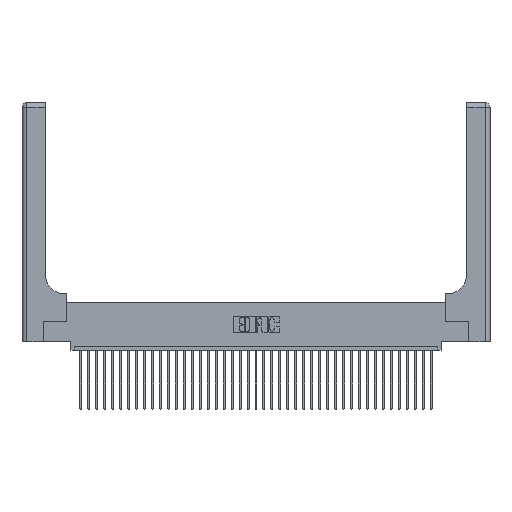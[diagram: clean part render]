
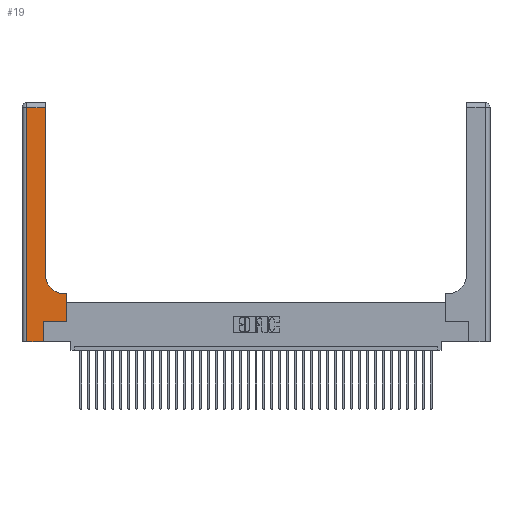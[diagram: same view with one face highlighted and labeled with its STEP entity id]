
A CAD part, top view. The second image highlights one B-rep face of the part: STEP entity #19.
In plain terms, the highlighted planar face has unit normal (0, 0, 1).
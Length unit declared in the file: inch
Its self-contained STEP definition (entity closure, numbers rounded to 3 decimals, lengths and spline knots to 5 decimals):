
#19 = ADVANCED_FACE ( 'NONE', ( #24024 ), #33489, .F. ) ;
#520 = CIRCLE ( 'NONE', #33592, 0.25 ) ;
#1753 = DIRECTION ( 'NONE',  ( 0., 1., 0. ) ) ;
#1925 = EDGE_CURVE ( 'NONE', #36288, #33440, #13026, .T. ) ;
#2226 = ORIENTED_EDGE ( 'NONE', *, *, #29808, .T. ) ;
#2275 = ORIENTED_EDGE ( 'NONE', *, *, #37258, .T. ) ;
#2957 = CARTESIAN_POINT ( 'NONE',  ( 0.2915, 2.94, 0.37 ) ) ;
#3867 = DIRECTION ( 'NONE',  ( 0., -1., 0. ) ) ;
#3986 = CARTESIAN_POINT ( 'NONE',  ( 0.06, 3., 0.37 ) ) ;
#4834 = ORIENTED_EDGE ( 'NONE', *, *, #14414, .T. ) ;
#4863 = ORIENTED_EDGE ( 'NONE', *, *, #14511, .T. ) ;
#5746 = CARTESIAN_POINT ( 'NONE',  ( 0.269, 0.25, 0.37 ) ) ;
#5756 = VERTEX_POINT ( 'NONE', #6281 ) ;
#5899 = LINE ( 'NONE', #3986, #30298 ) ;
#6281 = CARTESIAN_POINT ( 'NONE',  ( 0.269, 0.25, 0.37 ) ) ;
#6388 = LINE ( 'NONE', #12180, #35269 ) ;
#7393 = CARTESIAN_POINT ( 'NONE',  ( 0.269, 0., 0.37 ) ) ;
#7886 = DIRECTION ( 'NONE',  ( 0., 0., -1. ) ) ;
#9239 = LINE ( 'NONE', #35128, #25726 ) ;
#11020 = VERTEX_POINT ( 'NONE', #28412 ) ;
#11621 = VERTEX_POINT ( 'NONE', #22630 ) ;
#11805 = EDGE_LOOP ( 'NONE', ( #30937, #20879, #2226, #36488, #4834, #4863, #23236, #2275, #15407 ) ) ;
#12180 = CARTESIAN_POINT ( 'NONE',  ( 0.5585, 0.25, 0.37 ) ) ;
#12597 = DIRECTION ( 'NONE',  ( 1., 0., 0. ) ) ;
#13026 = LINE ( 'NONE', #31463, #26205 ) ;
#14183 = VERTEX_POINT ( 'NONE', #16431 ) ;
#14202 = DIRECTION ( 'NONE',  ( 0., 1., 0. ) ) ;
#14414 = EDGE_CURVE ( 'NONE', #34775, #5756, #9239, .T. ) ;
#14439 = DIRECTION ( 'NONE',  ( 1., 0., 0. ) ) ;
#14511 = EDGE_CURVE ( 'NONE', #5756, #14183, #35052, .T. ) ;
#14682 = EDGE_CURVE ( 'NONE', #14183, #11020, #6388, .T. ) ;
#15407 = ORIENTED_EDGE ( 'NONE', *, *, #32402, .T. ) ;
#15926 = LINE ( 'NONE', #20824, #18288 ) ;
#16431 = CARTESIAN_POINT ( 'NONE',  ( 0.5585, 0.25, 0.37 ) ) ;
#16763 = LINE ( 'NONE', #31006, #26140 ) ;
#16904 = CARTESIAN_POINT ( 'NONE',  ( 0.06, 2.94, 0.37 ) ) ;
#17067 = VERTEX_POINT ( 'NONE', #32489 ) ;
#17419 = VERTEX_POINT ( 'NONE', #30796 ) ;
#17866 = AXIS2_PLACEMENT_3D ( 'NONE', #38683, #7886, #23602 ) ;
#18288 = VECTOR ( 'NONE', #32971, 39.37008 ) ;
#18457 = EDGE_CURVE ( 'NONE', #17419, #36288, #15926, .T. ) ;
#19796 = EDGE_CURVE ( 'NONE', #17067, #34775, #16763, .T. ) ;
#20824 = CARTESIAN_POINT ( 'NONE',  ( 0.2915, 3., 0.37 ) ) ;
#20879 = ORIENTED_EDGE ( 'NONE', *, *, #1925, .T. ) ;
#21481 = CARTESIAN_POINT ( 'NONE',  ( 0.2915, 0.6, 0.37 ) ) ;
#22630 = CARTESIAN_POINT ( 'NONE',  ( 0.5415, 0.6, 0.37 ) ) ;
#23236 = ORIENTED_EDGE ( 'NONE', *, *, #14682, .T. ) ;
#23602 = DIRECTION ( 'NONE',  ( -1., 0., 0. ) ) ;
#23706 = VECTOR ( 'NONE', #30127, 39.37008 ) ;
#24024 = FACE_OUTER_BOUND ( 'NONE', #11805, .T. ) ;
#25132 = DIRECTION ( 'NONE',  ( 1., 0., 0. ) ) ;
#25726 = VECTOR ( 'NONE', #14202, 39.37008 ) ;
#26140 = VECTOR ( 'NONE', #25132, 39.37008 ) ;
#26205 = VECTOR ( 'NONE', #34717, 39.37008 ) ;
#27707 = DIRECTION ( 'NONE',  ( 0., 0., -1. ) ) ;
#28046 = VECTOR ( 'NONE', #14439, 39.37008 ) ;
#28412 = CARTESIAN_POINT ( 'NONE',  ( 0.5585, 0.6, 0.37 ) ) ;
#29808 = EDGE_CURVE ( 'NONE', #33440, #17067, #5899, .T. ) ;
#30127 = DIRECTION ( 'NONE',  ( -1., 0., 0. ) ) ;
#30298 = VECTOR ( 'NONE', #3867, 39.37008 ) ;
#30701 = CARTESIAN_POINT ( 'NONE',  ( 0.5415, 0.85, 0.37 ) ) ;
#30796 = CARTESIAN_POINT ( 'NONE',  ( 0.2915, 0.85, 0.37 ) ) ;
#30937 = ORIENTED_EDGE ( 'NONE', *, *, #18457, .T. ) ;
#31006 = CARTESIAN_POINT ( 'NONE',  ( 0., 0., 0.37 ) ) ;
#31463 = CARTESIAN_POINT ( 'NONE',  ( 0., 2.94, 0.37 ) ) ;
#32402 = EDGE_CURVE ( 'NONE', #11621, #17419, #520, .T. ) ;
#32489 = CARTESIAN_POINT ( 'NONE',  ( 0.06, 0., 0.37 ) ) ;
#32971 = DIRECTION ( 'NONE',  ( 0., 1., 0. ) ) ;
#33440 = VERTEX_POINT ( 'NONE', #16904 ) ;
#33489 = PLANE ( 'NONE',  #17866 ) ;
#33592 = AXIS2_PLACEMENT_3D ( 'NONE', #30701, #27707, #12597 ) ;
#34717 = DIRECTION ( 'NONE',  ( -1., 0., 0. ) ) ;
#34775 = VERTEX_POINT ( 'NONE', #7393 ) ;
#35052 = LINE ( 'NONE', #5746, #28046 ) ;
#35128 = CARTESIAN_POINT ( 'NONE',  ( 0.269, 0., 0.37 ) ) ;
#35269 = VECTOR ( 'NONE', #1753, 39.37008 ) ;
#36288 = VERTEX_POINT ( 'NONE', #2957 ) ;
#36488 = ORIENTED_EDGE ( 'NONE', *, *, #19796, .T. ) ;
#37258 = EDGE_CURVE ( 'NONE', #11020, #11621, #38601, .T. ) ;
#38601 = LINE ( 'NONE', #21481, #23706 ) ;
#38683 = CARTESIAN_POINT ( 'NONE',  ( 0., 3., 0.37 ) ) ;
